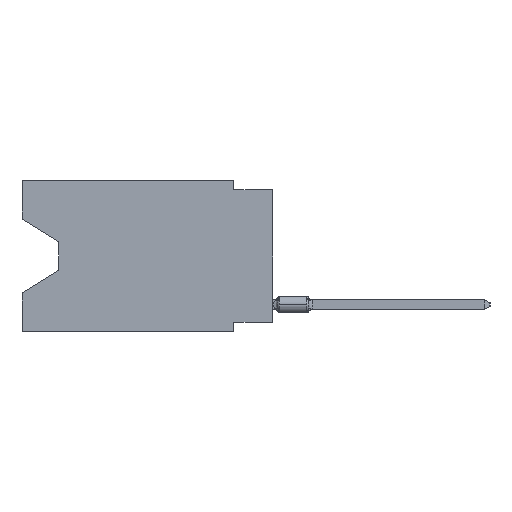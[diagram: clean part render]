
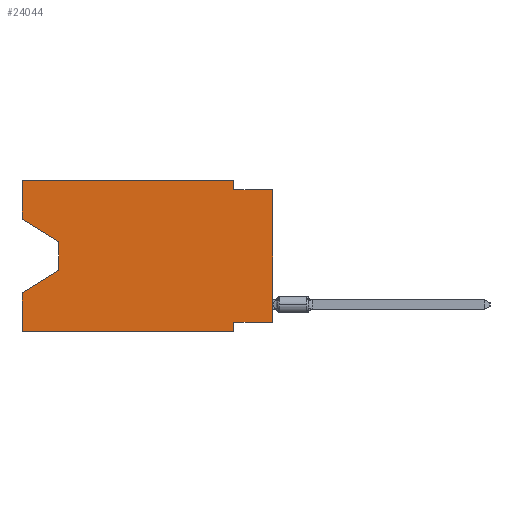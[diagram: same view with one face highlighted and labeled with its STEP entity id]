
A CAD part, left-side view. The second image highlights one B-rep face of the part: STEP entity #24044.
In plain terms, the highlighted planar face has unit normal (-1, 0, 0).
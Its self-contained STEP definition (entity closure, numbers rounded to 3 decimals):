
#98 = ORIENTED_EDGE ( 'NONE', *, *, #14175, .T. ) ;
#179 = AXIS2_PLACEMENT_3D ( 'NONE', #3294, #21350, #28160 ) ;
#704 = CARTESIAN_POINT ( 'NONE',  ( 0., 2.54, -9.271 ) ) ;
#721 = VECTOR ( 'NONE', #6891, 1000. ) ;
#768 = EDGE_CURVE ( 'NONE', #9897, #8218, #16407, .T. ) ;
#803 = CARTESIAN_POINT ( 'NONE',  ( 0., 13.97, -5.893 ) ) ;
#1447 = VECTOR ( 'NONE', #10697, 1000. ) ;
#2318 = CARTESIAN_POINT ( 'NONE',  ( 0., 0., -0.635 ) ) ;
#2359 = LINE ( 'NONE', #6376, #22876 ) ;
#2528 = VECTOR ( 'NONE', #7009, 1000. ) ;
#2581 = VERTEX_POINT ( 'NONE', #27485 ) ;
#2865 = DIRECTION ( 'NONE',  ( 0., 0.855, -0.519 ) ) ;
#3018 = LINE ( 'NONE', #12056, #2528 ) ;
#3125 = CARTESIAN_POINT ( 'NONE',  ( 0., 16.383, 0. ) ) ;
#3249 = VECTOR ( 'NONE', #21384, 1000. ) ;
#3261 = CARTESIAN_POINT ( 'NONE',  ( 0., 2.54, -9.906 ) ) ;
#3294 = CARTESIAN_POINT ( 'NONE',  ( 0., 16.383, 0. ) ) ;
#4431 = EDGE_CURVE ( 'NONE', #26690, #8218, #26190, .T. ) ;
#4586 = VERTEX_POINT ( 'NONE', #13164 ) ;
#4741 = VERTEX_POINT ( 'NONE', #21575 ) ;
#5360 = VECTOR ( 'NONE', #24501, 1000. ) ;
#5397 = DIRECTION ( 'NONE',  ( 0., 0., -1. ) ) ;
#5587 = CARTESIAN_POINT ( 'NONE',  ( 0., 16.383, -9.906 ) ) ;
#5844 = LINE ( 'NONE', #14449, #3249 ) ;
#6101 = CARTESIAN_POINT ( 'NONE',  ( 0., 16.383, 0. ) ) ;
#6376 = CARTESIAN_POINT ( 'NONE',  ( 0., 16.383, -2.546 ) ) ;
#6891 = DIRECTION ( 'NONE',  ( 0., 0., 1. ) ) ;
#6893 = CARTESIAN_POINT ( 'NONE',  ( 0., 16.383, 0. ) ) ;
#7009 = DIRECTION ( 'NONE',  ( 0., 1., 0. ) ) ;
#7347 = CARTESIAN_POINT ( 'NONE',  ( 0., 16.383, 0. ) ) ;
#7760 = EDGE_CURVE ( 'NONE', #12927, #4586, #10276, .T. ) ;
#8218 = VERTEX_POINT ( 'NONE', #17158 ) ;
#8877 = DIRECTION ( 'NONE',  ( 0., -1., 0. ) ) ;
#8907 = VERTEX_POINT ( 'NONE', #25069 ) ;
#9446 = ORIENTED_EDGE ( 'NONE', *, *, #28021, .T. ) ;
#9659 = VECTOR ( 'NONE', #14807, 1000. ) ;
#9897 = VERTEX_POINT ( 'NONE', #18292 ) ;
#10003 = ORIENTED_EDGE ( 'NONE', *, *, #22235, .T. ) ;
#10273 = ORIENTED_EDGE ( 'NONE', *, *, #768, .T. ) ;
#10276 = LINE ( 'NONE', #21223, #14803 ) ;
#10576 = VERTEX_POINT ( 'NONE', #6101 ) ;
#10697 = DIRECTION ( 'NONE',  ( 0., -1., 0. ) ) ;
#12053 = LINE ( 'NONE', #803, #22345 ) ;
#12056 = CARTESIAN_POINT ( 'NONE',  ( 0., 0., -9.271 ) ) ;
#12374 = VECTOR ( 'NONE', #14523, 1000. ) ;
#12927 = VERTEX_POINT ( 'NONE', #16829 ) ;
#13137 = ORIENTED_EDGE ( 'NONE', *, *, #28396, .F. ) ;
#13164 = CARTESIAN_POINT ( 'NONE',  ( 0., 2.54, -0.635 ) ) ;
#13447 = VERTEX_POINT ( 'NONE', #23677 ) ;
#13490 = LINE ( 'NONE', #7347, #19612 ) ;
#14175 = EDGE_CURVE ( 'NONE', #8907, #4741, #5844, .T. ) ;
#14449 = CARTESIAN_POINT ( 'NONE',  ( 0., 13.97, -4.013 ) ) ;
#14523 = DIRECTION ( 'NONE',  ( 0., 0., -1. ) ) ;
#14559 = FACE_OUTER_BOUND ( 'NONE', #20989, .T. ) ;
#14620 = DIRECTION ( 'NONE',  ( 0., -1., 0. ) ) ;
#14803 = VECTOR ( 'NONE', #5397, 1000. ) ;
#14807 = DIRECTION ( 'NONE',  ( 0., 0., 1. ) ) ;
#15488 = LINE ( 'NONE', #6893, #5360 ) ;
#15963 = EDGE_CURVE ( 'NONE', #4586, #17005, #19714, .T. ) ;
#16407 = LINE ( 'NONE', #5587, #24961 ) ;
#16829 = CARTESIAN_POINT ( 'NONE',  ( 0., 2.54, 0. ) ) ;
#17005 = VERTEX_POINT ( 'NONE', #2318 ) ;
#17158 = CARTESIAN_POINT ( 'NONE',  ( 0., 2.54, -9.906 ) ) ;
#17469 = ORIENTED_EDGE ( 'NONE', *, *, #7760, .F. ) ;
#17772 = DIRECTION ( 'NONE',  ( 0., -0.855, -0.519 ) ) ;
#18292 = CARTESIAN_POINT ( 'NONE',  ( 0., 16.383, -9.906 ) ) ;
#18846 = ORIENTED_EDGE ( 'NONE', *, *, #27336, .F. ) ;
#18901 = EDGE_CURVE ( 'NONE', #24484, #26690, #3018, .T. ) ;
#19167 = ORIENTED_EDGE ( 'NONE', *, *, #28902, .F. ) ;
#19612 = VECTOR ( 'NONE', #8877, 1000. ) ;
#19714 = LINE ( 'NONE', #28867, #1447 ) ;
#19830 = ORIENTED_EDGE ( 'NONE', *, *, #26096, .T. ) ;
#19948 = ORIENTED_EDGE ( 'NONE', *, *, #18901, .F. ) ;
#20952 = ORIENTED_EDGE ( 'NONE', *, *, #4431, .F. ) ;
#20959 = ORIENTED_EDGE ( 'NONE', *, *, #15963, .F. ) ;
#20989 = EDGE_LOOP ( 'NONE', ( #19830, #98, #9446, #19167, #10273, #20952, #19948, #10003, #20959, #17469, #18846, #13137 ) ) ;
#21223 = CARTESIAN_POINT ( 'NONE',  ( 0., 2.54, 0. ) ) ;
#21350 = DIRECTION ( 'NONE',  ( 1., 0., 0. ) ) ;
#21384 = DIRECTION ( 'NONE',  ( 0., 0., -1. ) ) ;
#21575 = CARTESIAN_POINT ( 'NONE',  ( 0., 13.97, -5.893 ) ) ;
#22235 = EDGE_CURVE ( 'NONE', #24484, #17005, #25225, .T. ) ;
#22345 = VECTOR ( 'NONE', #2865, 1000. ) ;
#22876 = VECTOR ( 'NONE', #17772, 1000. ) ;
#23574 = PLANE ( 'NONE',  #179 ) ;
#23677 = CARTESIAN_POINT ( 'NONE',  ( 0., 16.383, -7.36 ) ) ;
#24044 = ADVANCED_FACE ( 'NONE', ( #14559 ), #23574, .F. ) ;
#24224 = CARTESIAN_POINT ( 'NONE',  ( 0., 0., -9.271 ) ) ;
#24484 = VERTEX_POINT ( 'NONE', #24224 ) ;
#24501 = DIRECTION ( 'NONE',  ( 0., 0., 1. ) ) ;
#24961 = VECTOR ( 'NONE', #14620, 1000. ) ;
#25069 = CARTESIAN_POINT ( 'NONE',  ( 0., 13.97, -4.013 ) ) ;
#25225 = LINE ( 'NONE', #27158, #721 ) ;
#25903 = LINE ( 'NONE', #3125, #9659 ) ;
#26096 = EDGE_CURVE ( 'NONE', #2581, #8907, #2359, .T. ) ;
#26190 = LINE ( 'NONE', #3261, #12374 ) ;
#26690 = VERTEX_POINT ( 'NONE', #704 ) ;
#27158 = CARTESIAN_POINT ( 'NONE',  ( 0., 0., 0. ) ) ;
#27336 = EDGE_CURVE ( 'NONE', #10576, #12927, #13490, .T. ) ;
#27485 = CARTESIAN_POINT ( 'NONE',  ( 0., 16.383, -2.546 ) ) ;
#28021 = EDGE_CURVE ( 'NONE', #4741, #13447, #12053, .T. ) ;
#28160 = DIRECTION ( 'NONE',  ( 0., 0., -1. ) ) ;
#28396 = EDGE_CURVE ( 'NONE', #2581, #10576, #15488, .T. ) ;
#28867 = CARTESIAN_POINT ( 'NONE',  ( 0., 0., -0.635 ) ) ;
#28902 = EDGE_CURVE ( 'NONE', #9897, #13447, #25903, .T. ) ;
